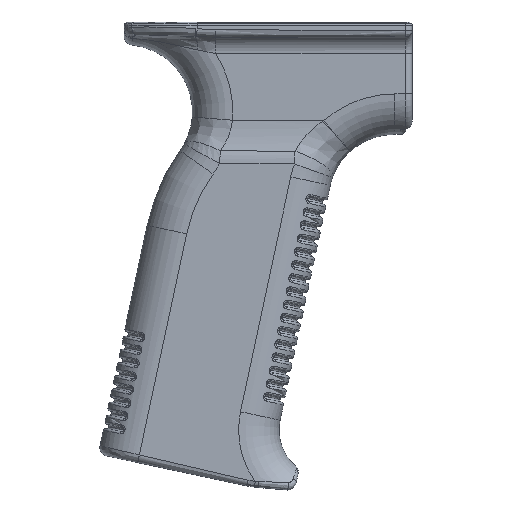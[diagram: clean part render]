
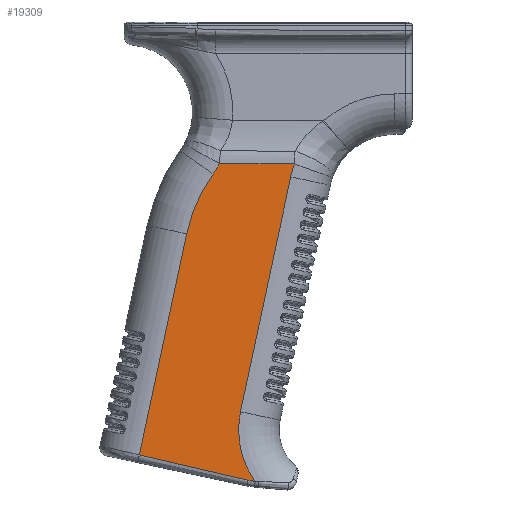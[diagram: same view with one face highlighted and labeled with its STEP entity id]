
A CAD part, front view. The second image highlights one B-rep face of the part: STEP entity #19309.
In plain terms, the highlighted planar face has unit normal (0, -1, 0).
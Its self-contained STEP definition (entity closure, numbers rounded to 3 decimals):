
#556=B_SPLINE_CURVE_WITH_KNOTS('',3,(#40616,#40617,#40618,#40619),
 .UNSPECIFIED.,.F.,.F.,(4,4),(3.901,4.066),
 .UNSPECIFIED.);
#558=B_SPLINE_CURVE_WITH_KNOTS('',3,(#40655,#40656,#40657,#40658),
 .UNSPECIFIED.,.F.,.F.,(4,4),(1.423,3.901),
 .UNSPECIFIED.);
#1365=LINE('',#27791,#2245);
#1671=LINE('',#33201,#2551);
#2014=LINE('',#40763,#2894);
#2245=VECTOR('',#22082,10.);
#2551=VECTOR('',#23552,10.);
#2894=VECTOR('',#26089,10.);
#3659=PLANE('',#21431);
#4647=FACE_OUTER_BOUND('',#5930,.T.);
#5930=EDGE_LOOP('',(#16648,#16649,#16650,#16651,#16652,#16653,#16654,#16655,
#16656));
#7374=CIRCLE('',#21424,19.5);
#7375=CIRCLE('',#21432,23.);
#7376=CIRCLE('',#21433,23.919);
#7377=CIRCLE('',#21434,36.);
#7682=VERTEX_POINT('',#27788);
#7683=VERTEX_POINT('',#27790);
#8255=VERTEX_POINT('',#33193);
#8256=VERTEX_POINT('',#33200);
#8858=VERTEX_POINT('',#40325);
#8862=VERTEX_POINT('',#40615);
#8867=VERTEX_POINT('',#40760);
#8868=VERTEX_POINT('',#40762);
#8869=VERTEX_POINT('',#40764);
#9431=EDGE_CURVE('',#7683,#7682,#1365,.T.);
#10311=EDGE_CURVE('',#8256,#8255,#1671,.T.);
#11493=EDGE_CURVE('',#8858,#7683,#7374,.T.);
#11503=EDGE_CURVE('',#8862,#8858,#556,.T.);
#11505=EDGE_CURVE('',#8255,#8862,#558,.T.);
#11516=EDGE_CURVE('',#7682,#8867,#7375,.T.);
#11517=EDGE_CURVE('',#8867,#8868,#2014,.T.);
#11518=EDGE_CURVE('',#8868,#8869,#7376,.T.);
#11519=EDGE_CURVE('',#8869,#8256,#7377,.T.);
#16648=ORIENTED_EDGE('',*,*,#9431,.T.);
#16649=ORIENTED_EDGE('',*,*,#11516,.T.);
#16650=ORIENTED_EDGE('',*,*,#11517,.T.);
#16651=ORIENTED_EDGE('',*,*,#11518,.T.);
#16652=ORIENTED_EDGE('',*,*,#11519,.T.);
#16653=ORIENTED_EDGE('',*,*,#10311,.T.);
#16654=ORIENTED_EDGE('',*,*,#11505,.T.);
#16655=ORIENTED_EDGE('',*,*,#11503,.T.);
#16656=ORIENTED_EDGE('',*,*,#11493,.T.);
#19309=ADVANCED_FACE('',(#4647),#3659,.F.);
#21424=AXIS2_PLACEMENT_3D('',#40326,#26065,#26066);
#21431=AXIS2_PLACEMENT_3D('',#40759,#26085,#26086);
#21432=AXIS2_PLACEMENT_3D('',#40761,#26087,#26088);
#21433=AXIS2_PLACEMENT_3D('',#40765,#26090,#26091);
#21434=AXIS2_PLACEMENT_3D('',#40766,#26092,#26093);
#22082=DIRECTION('',(0.209,0.,0.978));
#23552=DIRECTION('',(-0.209,0.,-0.978));
#26065=DIRECTION('center_axis',(0.,1.,0.));
#26066=DIRECTION('ref_axis',(-0.911,0.,-0.412));
#26085=DIRECTION('center_axis',(0.,1.,0.));
#26086=DIRECTION('ref_axis',(-1.,0.,0.));
#26087=DIRECTION('center_axis',(0.,1.,0.));
#26088=DIRECTION('ref_axis',(-0.924,0.,0.383));
#26089=DIRECTION('',(-1.,0.,0.006));
#26090=DIRECTION('center_axis',(0.,1.,0.));
#26091=DIRECTION('ref_axis',(0.669,0.,-0.743));
#26092=DIRECTION('center_axis',(0.,-1.,0.));
#26093=DIRECTION('ref_axis',(-0.93,0.,0.368));
#27788=CARTESIAN_POINT('',(22.103,-12.,-34.444));
#27790=CARTESIAN_POINT('',(10.928,-12.,-86.685));
#27791=CARTESIAN_POINT('',(20.167,-12.,-43.493));
#33193=CARTESIAN_POINT('',(-11.547,-12.,-96.278));
#33200=CARTESIAN_POINT('',(-1.03,-12.,-47.112));
#33201=CARTESIAN_POINT('',(-7.107,-12.,-75.523));
#40325=CARTESIAN_POINT('',(14.198,-12.,-102.195));
#40326=CARTESIAN_POINT('Origin',(29.997,-12.,-90.764));
#40615=CARTESIAN_POINT('',(12.583,-12.,-101.893));
#40616=CARTESIAN_POINT('Ctrl Pts',(12.583,-12.,-101.893));
#40617=CARTESIAN_POINT('Ctrl Pts',(13.116,-12.,-102.017));
#40618=CARTESIAN_POINT('Ctrl Pts',(13.655,-12.,-102.118));
#40619=CARTESIAN_POINT('Ctrl Pts',(14.198,-12.,-102.195));
#40655=CARTESIAN_POINT('Ctrl Pts',(-11.547,-12.,-96.278));
#40656=CARTESIAN_POINT('Ctrl Pts',(-3.492,-12.,-98.152));
#40657=CARTESIAN_POINT('Ctrl Pts',(4.539,-12.,-100.021));
#40658=CARTESIAN_POINT('Ctrl Pts',(12.583,-12.,-101.893));
#40759=CARTESIAN_POINT('Origin',(14.194,-12.,-53.522));
#40760=CARTESIAN_POINT('',(22.913,-12.,-31.579));
#40761=CARTESIAN_POINT('Origin',(44.594,-12.,-39.255));
#40762=CARTESIAN_POINT('',(6.274,-12.,-31.48));
#40763=CARTESIAN_POINT('',(5.892,-12.,-31.477));
#40764=CARTESIAN_POINT('',(4.815,-12.,-33.807));
#40765=CARTESIAN_POINT('Origin',(-14.69,-12.,-19.964));
#40766=CARTESIAN_POINT('Origin',(34.173,-12.,-54.642));
